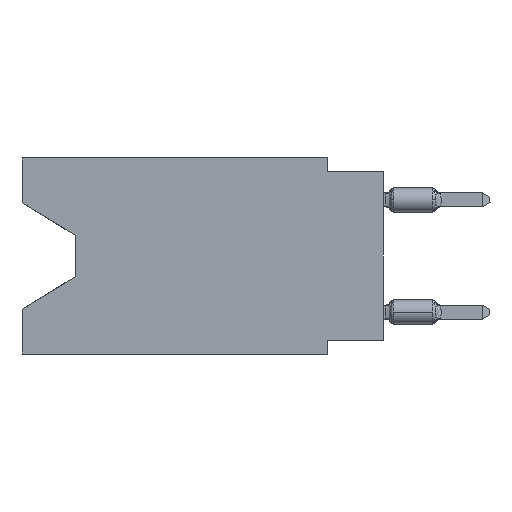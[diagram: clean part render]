
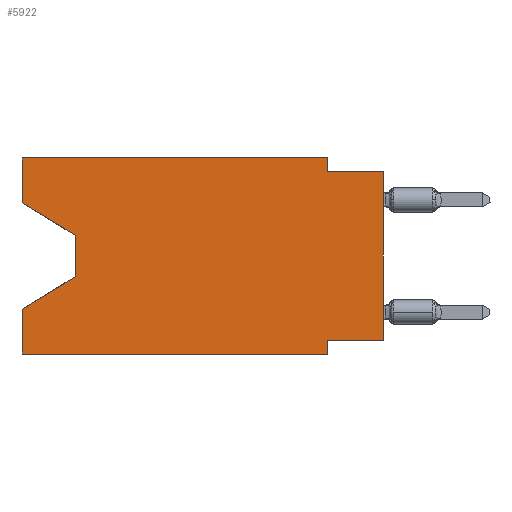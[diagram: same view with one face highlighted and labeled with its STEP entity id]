
A CAD part, left-side view. The second image highlights one B-rep face of the part: STEP entity #5922.
In plain terms, the highlighted planar face has unit normal (-1, 0, 0).
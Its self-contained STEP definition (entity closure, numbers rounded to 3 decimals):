
#154 = DIRECTION ( 'NONE',  ( 0., 0., -1. ) ) ;
#1344 = CARTESIAN_POINT ( 'NONE',  ( 0., 16.383, -8.89 ) ) ;
#1493 = VECTOR ( 'NONE', #45475, 1000. ) ;
#1604 = VECTOR ( 'NONE', #33093, 1000. ) ;
#1623 = EDGE_CURVE ( 'NONE', #14177, #37192, #36887, .T. ) ;
#1827 = AXIS2_PLACEMENT_3D ( 'NONE', #8430, #15994, #34209 ) ;
#2956 = VECTOR ( 'NONE', #29829, 1000. ) ;
#3290 = LINE ( 'NONE', #31949, #21205 ) ;
#3645 = VERTEX_POINT ( 'NONE', #41236 ) ;
#3990 = CARTESIAN_POINT ( 'NONE',  ( 0., 2.54, -8.255 ) ) ;
#4788 = LINE ( 'NONE', #27029, #43004 ) ;
#5922 = ADVANCED_FACE ( 'NONE', ( #41301 ), #26654, .F. ) ;
#6488 = CARTESIAN_POINT ( 'NONE',  ( 0., 16.383, 0. ) ) ;
#6819 = CARTESIAN_POINT ( 'NONE',  ( 0., 16.383, -6.852 ) ) ;
#7012 = EDGE_CURVE ( 'NONE', #14177, #35882, #30002, .T. ) ;
#7951 = CARTESIAN_POINT ( 'NONE',  ( 0., 2.54, -8.89 ) ) ;
#8054 = LINE ( 'NONE', #22964, #2956 ) ;
#8430 = CARTESIAN_POINT ( 'NONE',  ( 0., 16.383, 0. ) ) ;
#8931 = ORIENTED_EDGE ( 'NONE', *, *, #7012, .T. ) ;
#9056 = DIRECTION ( 'NONE',  ( 0., 0., -1. ) ) ;
#9133 = CARTESIAN_POINT ( 'NONE',  ( 0., 0., -8.255 ) ) ;
#9282 = VERTEX_POINT ( 'NONE', #11681 ) ;
#9632 = ORIENTED_EDGE ( 'NONE', *, *, #20539, .F. ) ;
#9662 = ORIENTED_EDGE ( 'NONE', *, *, #35529, .T. ) ;
#9800 = VECTOR ( 'NONE', #44485, 1000. ) ;
#10400 = ORIENTED_EDGE ( 'NONE', *, *, #31839, .T. ) ;
#10735 = VECTOR ( 'NONE', #30592, 1000. ) ;
#11438 = ORIENTED_EDGE ( 'NONE', *, *, #26619, .F. ) ;
#11627 = CARTESIAN_POINT ( 'NONE',  ( 0., 16.383, 0. ) ) ;
#11681 = CARTESIAN_POINT ( 'NONE',  ( 0., 2.54, 0. ) ) ;
#11766 = EDGE_CURVE ( 'NONE', #20027, #9282, #37621, .T. ) ;
#11810 = EDGE_CURVE ( 'NONE', #25703, #11990, #8054, .T. ) ;
#11990 = VERTEX_POINT ( 'NONE', #3990 ) ;
#13808 = CARTESIAN_POINT ( 'NONE',  ( 0., 13.97, -5.385 ) ) ;
#14177 = VERTEX_POINT ( 'NONE', #26571 ) ;
#15034 = ORIENTED_EDGE ( 'NONE', *, *, #32549, .T. ) ;
#15366 = CARTESIAN_POINT ( 'NONE',  ( 0., 16.383, 0. ) ) ;
#15450 = CARTESIAN_POINT ( 'NONE',  ( 0., 13.97, -3.505 ) ) ;
#15994 = DIRECTION ( 'NONE',  ( 1., 0., 0. ) ) ;
#16166 = LINE ( 'NONE', #33901, #10735 ) ;
#16463 = EDGE_CURVE ( 'NONE', #11990, #35882, #40375, .T. ) ;
#17437 = VECTOR ( 'NONE', #24484, 1000. ) ;
#17648 = ORIENTED_EDGE ( 'NONE', *, *, #16463, .F. ) ;
#19371 = CARTESIAN_POINT ( 'NONE',  ( 0., 2.54, -8.89 ) ) ;
#19749 = CARTESIAN_POINT ( 'NONE',  ( 0., 16.383, 0. ) ) ;
#20027 = VERTEX_POINT ( 'NONE', #19749 ) ;
#20366 = LINE ( 'NONE', #22988, #1493 ) ;
#20539 = EDGE_CURVE ( 'NONE', #9282, #41547, #4788, .T. ) ;
#21205 = VECTOR ( 'NONE', #35727, 1000. ) ;
#22310 = CARTESIAN_POINT ( 'NONE',  ( 0., 2.54, -0.635 ) ) ;
#22933 = DIRECTION ( 'NONE',  ( 0., 0., 1. ) ) ;
#22964 = CARTESIAN_POINT ( 'NONE',  ( 0., 0., -8.255 ) ) ;
#22988 = CARTESIAN_POINT ( 'NONE',  ( 0., 13.97, -5.385 ) ) ;
#24484 = DIRECTION ( 'NONE',  ( 0., 0., 1. ) ) ;
#25669 = VERTEX_POINT ( 'NONE', #29951 ) ;
#25703 = VERTEX_POINT ( 'NONE', #9133 ) ;
#26571 = CARTESIAN_POINT ( 'NONE',  ( 0., 16.383, -8.89 ) ) ;
#26619 = EDGE_CURVE ( 'NONE', #3645, #20027, #42232, .T. ) ;
#26654 = PLANE ( 'NONE',  #1827 ) ;
#26813 = ORIENTED_EDGE ( 'NONE', *, *, #1623, .F. ) ;
#27029 = CARTESIAN_POINT ( 'NONE',  ( 0., 2.54, 0. ) ) ;
#27172 = VECTOR ( 'NONE', #41227, 1000. ) ;
#29829 = DIRECTION ( 'NONE',  ( 0., 1., 0. ) ) ;
#29951 = CARTESIAN_POINT ( 'NONE',  ( 0., 0., -0.635 ) ) ;
#30002 = LINE ( 'NONE', #1344, #1604 ) ;
#30592 = DIRECTION ( 'NONE',  ( 0., -0.855, -0.519 ) ) ;
#30602 = DIRECTION ( 'NONE',  ( 0., -1., 0. ) ) ;
#30694 = VECTOR ( 'NONE', #154, 1000. ) ;
#31839 = EDGE_CURVE ( 'NONE', #39094, #35241, #33894, .T. ) ;
#31949 = CARTESIAN_POINT ( 'NONE',  ( 0., 0., 0. ) ) ;
#32549 = EDGE_CURVE ( 'NONE', #25703, #25669, #3290, .T. ) ;
#33093 = DIRECTION ( 'NONE',  ( 0., -1., 0. ) ) ;
#33593 = ORIENTED_EDGE ( 'NONE', *, *, #11810, .F. ) ;
#33894 = LINE ( 'NONE', #15450, #27172 ) ;
#33901 = CARTESIAN_POINT ( 'NONE',  ( 0., 16.383, -2.038 ) ) ;
#34209 = DIRECTION ( 'NONE',  ( 0., 0., -1. ) ) ;
#35140 = EDGE_CURVE ( 'NONE', #41547, #25669, #44816, .T. ) ;
#35241 = VERTEX_POINT ( 'NONE', #13808 ) ;
#35529 = EDGE_CURVE ( 'NONE', #35241, #37192, #20366, .T. ) ;
#35727 = DIRECTION ( 'NONE',  ( 0., 0., 1. ) ) ;
#35882 = VERTEX_POINT ( 'NONE', #19371 ) ;
#36183 = EDGE_LOOP ( 'NONE', ( #44995, #10400, #9662, #26813, #8931, #17648, #33593, #15034, #36558, #9632, #37625, #11438 ) ) ;
#36461 = CARTESIAN_POINT ( 'NONE',  ( 0., 13.97, -3.505 ) ) ;
#36558 = ORIENTED_EDGE ( 'NONE', *, *, #35140, .F. ) ;
#36764 = VECTOR ( 'NONE', #22933, 1000. ) ;
#36887 = LINE ( 'NONE', #15366, #36764 ) ;
#37192 = VERTEX_POINT ( 'NONE', #6819 ) ;
#37621 = LINE ( 'NONE', #11627, #9800 ) ;
#37625 = ORIENTED_EDGE ( 'NONE', *, *, #11766, .F. ) ;
#38399 = CARTESIAN_POINT ( 'NONE',  ( 0., 0., -0.635 ) ) ;
#39094 = VERTEX_POINT ( 'NONE', #36461 ) ;
#40375 = LINE ( 'NONE', #7951, #30694 ) ;
#41227 = DIRECTION ( 'NONE',  ( 0., 0., -1. ) ) ;
#41236 = CARTESIAN_POINT ( 'NONE',  ( 0., 16.383, -2.038 ) ) ;
#41301 = FACE_OUTER_BOUND ( 'NONE', #36183, .T. ) ;
#41547 = VERTEX_POINT ( 'NONE', #22310 ) ;
#42232 = LINE ( 'NONE', #6488, #17437 ) ;
#43004 = VECTOR ( 'NONE', #9056, 1000. ) ;
#44485 = DIRECTION ( 'NONE',  ( 0., -1., 0. ) ) ;
#44542 = VECTOR ( 'NONE', #30602, 1000. ) ;
#44816 = LINE ( 'NONE', #38399, #44542 ) ;
#44995 = ORIENTED_EDGE ( 'NONE', *, *, #45311, .T. ) ;
#45311 = EDGE_CURVE ( 'NONE', #3645, #39094, #16166, .T. ) ;
#45475 = DIRECTION ( 'NONE',  ( 0., 0.855, -0.519 ) ) ;
